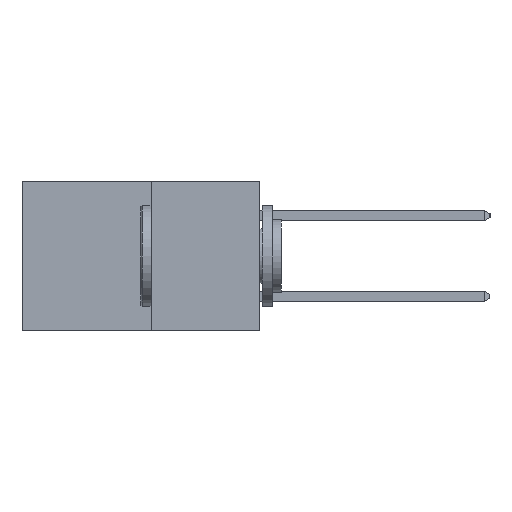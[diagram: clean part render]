
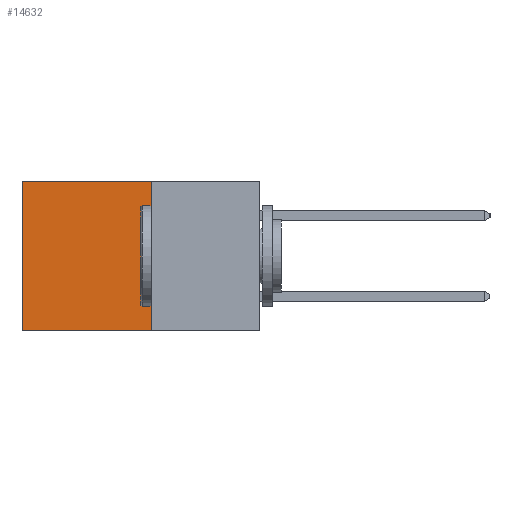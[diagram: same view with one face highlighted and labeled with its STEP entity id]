
A CAD part, left-side view. The second image highlights one B-rep face of the part: STEP entity #14632.
In plain terms, the highlighted planar face has unit normal (-1, 0, 0).
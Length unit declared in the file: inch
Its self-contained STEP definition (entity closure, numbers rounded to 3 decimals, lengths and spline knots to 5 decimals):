
#134 = EDGE_CURVE ( 'NONE', #1343, #7722, #15906, .T. ) ;
#408 = DIRECTION ( 'NONE',  ( 0., 1., 0. ) ) ;
#693 = DIRECTION ( 'NONE',  ( 1., 0., 0. ) ) ;
#1175 = LINE ( 'NONE', #4406, #19156 ) ;
#1343 = VERTEX_POINT ( 'NONE', #1346 ) ;
#1346 = CARTESIAN_POINT ( 'NONE',  ( 0.277, 0.27, 0. ) ) ;
#1878 = VECTOR ( 'NONE', #7318, 39.37008 ) ;
#2289 = VERTEX_POINT ( 'NONE', #20465 ) ;
#2305 = AXIS2_PLACEMENT_3D ( 'NONE', #11300, #693, #13030 ) ;
#2683 = VECTOR ( 'NONE', #14098, 39.37008 ) ;
#3222 = ORIENTED_EDGE ( 'NONE', *, *, #13917, .T. ) ;
#4079 = CARTESIAN_POINT ( 'NONE',  ( 0.277, 0.27, -0.37 ) ) ;
#4406 = CARTESIAN_POINT ( 'NONE',  ( 0.277, 0.27, -0.37 ) ) ;
#4409 = DIRECTION ( 'NONE',  ( 0., 1., 0. ) ) ;
#5158 = EDGE_CURVE ( 'NONE', #7722, #2289, #1175, .T. ) ;
#6308 = CARTESIAN_POINT ( 'NONE',  ( 0.277, 0.59, 0. ) ) ;
#7318 = DIRECTION ( 'NONE',  ( 0., 0., -1. ) ) ;
#7722 = VERTEX_POINT ( 'NONE', #17481 ) ;
#7764 = PLANE ( 'NONE',  #2305 ) ;
#9594 = ORIENTED_EDGE ( 'NONE', *, *, #5158, .F. ) ;
#10646 = CARTESIAN_POINT ( 'NONE',  ( 0.277, 0.59, -0.37 ) ) ;
#11300 = CARTESIAN_POINT ( 'NONE',  ( 0.277, 0.27, -0.37 ) ) ;
#11528 = LINE ( 'NONE', #19544, #15037 ) ;
#12623 = EDGE_LOOP ( 'NONE', ( #22134, #9594, #17956, #3222 ) ) ;
#13030 = DIRECTION ( 'NONE',  ( 0., 0., -1. ) ) ;
#13917 = EDGE_CURVE ( 'NONE', #1343, #18744, #11528, .T. ) ;
#14098 = DIRECTION ( 'NONE',  ( 0., 0., -1. ) ) ;
#14632 = ADVANCED_FACE ( 'NONE', ( #19547 ), #7764, .F. ) ;
#15037 = VECTOR ( 'NONE', #408, 39.37008 ) ;
#15906 = LINE ( 'NONE', #4079, #1878 ) ;
#17481 = CARTESIAN_POINT ( 'NONE',  ( 0.277, 0.27, -0.37 ) ) ;
#17725 = LINE ( 'NONE', #10646, #2683 ) ;
#17956 = ORIENTED_EDGE ( 'NONE', *, *, #134, .F. ) ;
#18744 = VERTEX_POINT ( 'NONE', #6308 ) ;
#19048 = EDGE_CURVE ( 'NONE', #18744, #2289, #17725, .T. ) ;
#19156 = VECTOR ( 'NONE', #4409, 39.37008 ) ;
#19544 = CARTESIAN_POINT ( 'NONE',  ( 0.277, 0.27, 0. ) ) ;
#19547 = FACE_OUTER_BOUND ( 'NONE', #12623, .T. ) ;
#20465 = CARTESIAN_POINT ( 'NONE',  ( 0.277, 0.59, -0.37 ) ) ;
#22134 = ORIENTED_EDGE ( 'NONE', *, *, #19048, .T. ) ;
